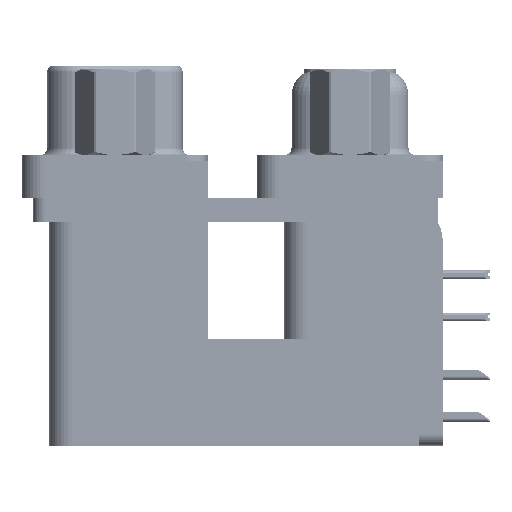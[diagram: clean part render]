
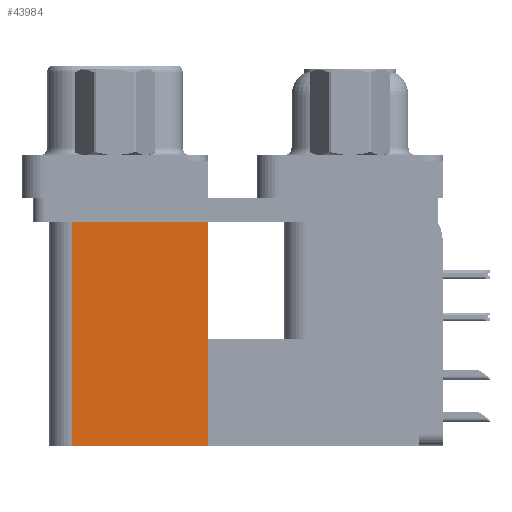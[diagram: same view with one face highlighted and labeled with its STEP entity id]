
A CAD part, left-side view. The second image highlights one B-rep face of the part: STEP entity #43984.
In plain terms, the highlighted planar face has unit normal (-1, 0, 0).
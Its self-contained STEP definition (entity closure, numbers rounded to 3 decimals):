
#582 = CARTESIAN_POINT ( 'NONE',  ( 3.7, 18.8, -2.5 ) ) ;
#1048 = VERTEX_POINT ( 'NONE', #59343 ) ;
#4714 = ORIENTED_EDGE ( 'NONE', *, *, #17129, .F. ) ;
#5910 = LINE ( 'NONE', #46955, #24068 ) ;
#8578 = LINE ( 'NONE', #39954, #33161 ) ;
#12528 = EDGE_CURVE ( 'NONE', #1048, #56804, #8578, .T. ) ;
#15923 = VERTEX_POINT ( 'NONE', #25720 ) ;
#17129 = EDGE_CURVE ( 'NONE', #1048, #15923, #19060, .T. ) ;
#19060 = LINE ( 'NONE', #27521, #26797 ) ;
#20512 = ORIENTED_EDGE ( 'NONE', *, *, #12528, .T. ) ;
#20631 = PLANE ( 'NONE',  #46458 ) ;
#24068 = VECTOR ( 'NONE', #50108, 1000. ) ;
#25144 = FACE_OUTER_BOUND ( 'NONE', #28445, .T. ) ;
#25457 = DIRECTION ( 'NONE',  ( 1., 0., 0. ) ) ;
#25720 = CARTESIAN_POINT ( 'NONE',  ( 3.7, 18.8, -19.2 ) ) ;
#26675 = EDGE_CURVE ( 'NONE', #15923, #49292, #56818, .T. ) ;
#26797 = VECTOR ( 'NONE', #36865, 1000. ) ;
#27521 = CARTESIAN_POINT ( 'NONE',  ( 3.7, 9.6, -19.2 ) ) ;
#28445 = EDGE_LOOP ( 'NONE', ( #41864, #44751, #4714, #20512 ) ) ;
#33161 = VECTOR ( 'NONE', #40552, 1000. ) ;
#33747 = CARTESIAN_POINT ( 'NONE',  ( 3.7, 9.6, -2.5 ) ) ;
#36865 = DIRECTION ( 'NONE',  ( 0., 1., 0. ) ) ;
#38739 = EDGE_CURVE ( 'NONE', #56804, #49292, #5910, .T. ) ;
#39954 = CARTESIAN_POINT ( 'NONE',  ( 3.7, 9.6, -19.2 ) ) ;
#40552 = DIRECTION ( 'NONE',  ( 0., 0., 1. ) ) ;
#41864 = ORIENTED_EDGE ( 'NONE', *, *, #38739, .T. ) ;
#43858 = CARTESIAN_POINT ( 'NONE',  ( 3.7, 9.6, -19.2 ) ) ;
#43984 = ADVANCED_FACE ( 'NONE', ( #25144 ), #20631, .F. ) ;
#44751 = ORIENTED_EDGE ( 'NONE', *, *, #26675, .F. ) ;
#46458 = AXIS2_PLACEMENT_3D ( 'NONE', #43858, #25457, #53244 ) ;
#46955 = CARTESIAN_POINT ( 'NONE',  ( 3.7, 9.6, -2.5 ) ) ;
#49292 = VERTEX_POINT ( 'NONE', #582 ) ;
#50108 = DIRECTION ( 'NONE',  ( 0., 1., 0. ) ) ;
#52873 = DIRECTION ( 'NONE',  ( 0., 0., 1. ) ) ;
#53244 = DIRECTION ( 'NONE',  ( 0., 0., -1. ) ) ;
#54925 = VECTOR ( 'NONE', #52873, 1000. ) ;
#56520 = CARTESIAN_POINT ( 'NONE',  ( 3.7, 18.8, -19.2 ) ) ;
#56804 = VERTEX_POINT ( 'NONE', #33747 ) ;
#56818 = LINE ( 'NONE', #56520, #54925 ) ;
#59343 = CARTESIAN_POINT ( 'NONE',  ( 3.7, 9.6, -19.2 ) ) ;
